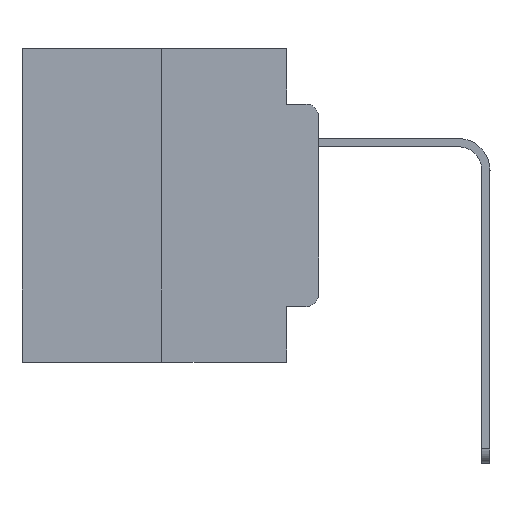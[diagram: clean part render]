
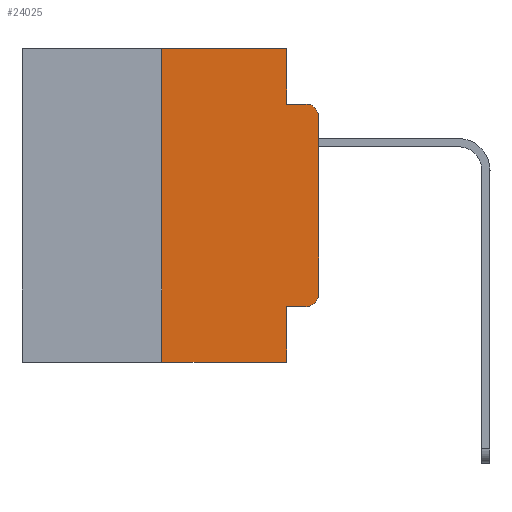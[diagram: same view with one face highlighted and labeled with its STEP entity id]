
A CAD part, left-side view. The second image highlights one B-rep face of the part: STEP entity #24025.
In plain terms, the highlighted planar face has unit normal (-1, 0, 0).
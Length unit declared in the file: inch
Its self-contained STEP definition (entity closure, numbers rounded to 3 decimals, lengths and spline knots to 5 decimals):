
#496 = CARTESIAN_POINT ( 'NONE',  ( 0., 0., 0. ) ) ;
#1041 = VECTOR ( 'NONE', #25214, 39.37008 ) ;
#1628 = ORIENTED_EDGE ( 'NONE', *, *, #19740, .T. ) ;
#1661 = LINE ( 'NONE', #17277, #1041 ) ;
#2009 = LINE ( 'NONE', #8357, #13249 ) ;
#2324 = ORIENTED_EDGE ( 'NONE', *, *, #22944, .F. ) ;
#2727 = ORIENTED_EDGE ( 'NONE', *, *, #18940, .F. ) ;
#3206 = CARTESIAN_POINT ( 'NONE',  ( 0., 0.051, 0. ) ) ;
#4451 = VERTEX_POINT ( 'NONE', #25840 ) ;
#4845 = AXIS2_PLACEMENT_3D ( 'NONE', #7198, #13141, #25255 ) ;
#5910 = VERTEX_POINT ( 'NONE', #16225 ) ;
#6849 = CARTESIAN_POINT ( 'NONE',  ( 0., 0.051, 0. ) ) ;
#7042 = CARTESIAN_POINT ( 'NONE',  ( 0., 0.051, 0. ) ) ;
#7198 = CARTESIAN_POINT ( 'NONE',  ( 0., 0.473, 0. ) ) ;
#7585 = EDGE_CURVE ( 'NONE', #23035, #22550, #1661, .T. ) ;
#8357 = CARTESIAN_POINT ( 'NONE',  ( 0., 0.051, -0.4115 ) ) ;
#8419 = CARTESIAN_POINT ( 'NONE',  ( 0., 0.02, -0.4115 ) ) ;
#8649 = VERTEX_POINT ( 'NONE', #20987 ) ;
#8701 = CARTESIAN_POINT ( 'NONE',  ( 0., 0.25, 0. ) ) ;
#9038 = CARTESIAN_POINT ( 'NONE',  ( 0., 0.473, 0. ) ) ;
#9144 = CARTESIAN_POINT ( 'NONE',  ( 0., 0.02, -0.3915 ) ) ;
#9314 = LINE ( 'NONE', #15750, #15555 ) ;
#9631 = AXIS2_PLACEMENT_3D ( 'NONE', #21420, #19182, #13490 ) ;
#9644 = DIRECTION ( 'NONE',  ( 0., -1., 0. ) ) ;
#9858 = LINE ( 'NONE', #496, #19861 ) ;
#10239 = VERTEX_POINT ( 'NONE', #13539 ) ;
#10766 = VECTOR ( 'NONE', #19175, 39.37008 ) ;
#10898 = CARTESIAN_POINT ( 'NONE',  ( 0., 0.02, -0.0885 ) ) ;
#11160 = DIRECTION ( 'NONE',  ( 0., 0., -1. ) ) ;
#11311 = EDGE_CURVE ( 'NONE', #4451, #12285, #19536, .T. ) ;
#11449 = VERTEX_POINT ( 'NONE', #13756 ) ;
#11983 = EDGE_CURVE ( 'NONE', #11449, #21370, #2009, .T. ) ;
#12227 = EDGE_CURVE ( 'NONE', #24365, #8649, #15113, .T. ) ;
#12285 = VERTEX_POINT ( 'NONE', #10898 ) ;
#12378 = DIRECTION ( 'NONE',  ( 0., -1., 0. ) ) ;
#13008 = FACE_OUTER_BOUND ( 'NONE', #16861, .T. ) ;
#13141 = DIRECTION ( 'NONE',  ( 1., 0., 0. ) ) ;
#13204 = ORIENTED_EDGE ( 'NONE', *, *, #11311, .T. ) ;
#13249 = VECTOR ( 'NONE', #12378, 39.37008 ) ;
#13490 = DIRECTION ( 'NONE',  ( 0., 0., -1. ) ) ;
#13539 = CARTESIAN_POINT ( 'NONE',  ( 0., 0.051, -0.5 ) ) ;
#13756 = CARTESIAN_POINT ( 'NONE',  ( 0., 0.051, -0.4115 ) ) ;
#13757 = CIRCLE ( 'NONE', #18991, 0.02 ) ;
#13853 = VECTOR ( 'NONE', #11160, 39.37008 ) ;
#13998 = VECTOR ( 'NONE', #17323, 39.37008 ) ;
#14134 = ORIENTED_EDGE ( 'NONE', *, *, #19041, .T. ) ;
#14979 = PLANE ( 'NONE',  #4845 ) ;
#15113 = LINE ( 'NONE', #7042, #13853 ) ;
#15318 = CARTESIAN_POINT ( 'NONE',  ( 0., 0.473, -0.5 ) ) ;
#15555 = VECTOR ( 'NONE', #9644, 39.37008 ) ;
#15739 = LINE ( 'NONE', #9038, #10766 ) ;
#15750 = CARTESIAN_POINT ( 'NONE',  ( 0., 0.051, -0.0885 ) ) ;
#15786 = EDGE_CURVE ( 'NONE', #5910, #4451, #9858, .T. ) ;
#16225 = CARTESIAN_POINT ( 'NONE',  ( 0., 0., -0.3915 ) ) ;
#16861 = EDGE_LOOP ( 'NONE', ( #20070, #13204, #2324, #23258, #24753, #20258, #1628, #2727, #17861, #14134 ) ) ;
#17003 = DIRECTION ( 'NONE',  ( -1., 0., 0. ) ) ;
#17277 = CARTESIAN_POINT ( 'NONE',  ( 0., 0.25, 0. ) ) ;
#17323 = DIRECTION ( 'NONE',  ( 0., -1., 0. ) ) ;
#17794 = LINE ( 'NONE', #3206, #22478 ) ;
#17861 = ORIENTED_EDGE ( 'NONE', *, *, #11983, .T. ) ;
#18700 = LINE ( 'NONE', #15318, #13998 ) ;
#18940 = EDGE_CURVE ( 'NONE', #11449, #10239, #17794, .T. ) ;
#18991 = AXIS2_PLACEMENT_3D ( 'NONE', #9144, #17003, #21276 ) ;
#19041 = EDGE_CURVE ( 'NONE', #21370, #5910, #13757, .T. ) ;
#19175 = DIRECTION ( 'NONE',  ( 0., -1., 0. ) ) ;
#19182 = DIRECTION ( 'NONE',  ( -1., 0., 0. ) ) ;
#19536 = CIRCLE ( 'NONE', #9631, 0.02 ) ;
#19740 = EDGE_CURVE ( 'NONE', #23035, #10239, #18700, .T. ) ;
#19861 = VECTOR ( 'NONE', #24642, 39.37008 ) ;
#20070 = ORIENTED_EDGE ( 'NONE', *, *, #15786, .T. ) ;
#20258 = ORIENTED_EDGE ( 'NONE', *, *, #7585, .F. ) ;
#20987 = CARTESIAN_POINT ( 'NONE',  ( 0., 0.051, -0.0885 ) ) ;
#21023 = DIRECTION ( 'NONE',  ( 0., 0., -1. ) ) ;
#21276 = DIRECTION ( 'NONE',  ( 0., 0., -1. ) ) ;
#21370 = VERTEX_POINT ( 'NONE', #8419 ) ;
#21420 = CARTESIAN_POINT ( 'NONE',  ( 0., 0.02, -0.1085 ) ) ;
#21587 = CARTESIAN_POINT ( 'NONE',  ( 0., 0.25, -0.5 ) ) ;
#22478 = VECTOR ( 'NONE', #21023, 39.37008 ) ;
#22550 = VERTEX_POINT ( 'NONE', #8701 ) ;
#22944 = EDGE_CURVE ( 'NONE', #8649, #12285, #9314, .T. ) ;
#23035 = VERTEX_POINT ( 'NONE', #21587 ) ;
#23258 = ORIENTED_EDGE ( 'NONE', *, *, #12227, .F. ) ;
#24025 = ADVANCED_FACE ( 'NONE', ( #13008 ), #14979, .F. ) ;
#24365 = VERTEX_POINT ( 'NONE', #6849 ) ;
#24642 = DIRECTION ( 'NONE',  ( 0., 0., 1. ) ) ;
#24753 = ORIENTED_EDGE ( 'NONE', *, *, #25725, .F. ) ;
#25214 = DIRECTION ( 'NONE',  ( 0., 0., 1. ) ) ;
#25255 = DIRECTION ( 'NONE',  ( 0., 0., -1. ) ) ;
#25725 = EDGE_CURVE ( 'NONE', #22550, #24365, #15739, .T. ) ;
#25840 = CARTESIAN_POINT ( 'NONE',  ( 0., 0., -0.1085 ) ) ;
